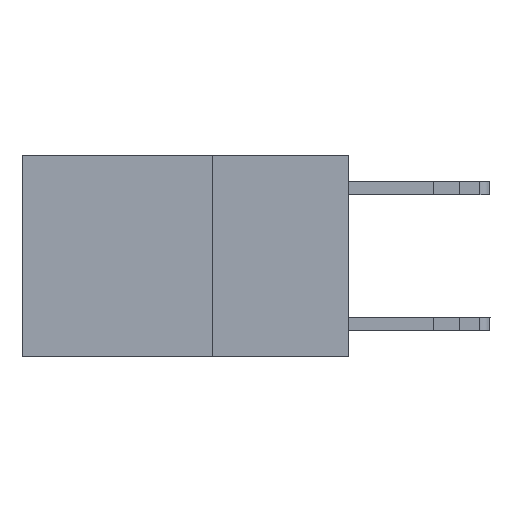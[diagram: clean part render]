
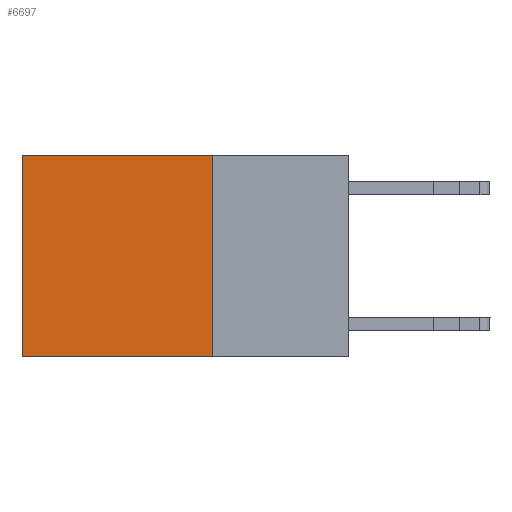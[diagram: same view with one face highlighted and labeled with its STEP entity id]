
A CAD part, left-side view. The second image highlights one B-rep face of the part: STEP entity #6697.
In plain terms, the highlighted planar face has unit normal (-1, 0, 0).
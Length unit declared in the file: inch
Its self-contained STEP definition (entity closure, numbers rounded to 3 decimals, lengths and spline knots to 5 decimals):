
#104 = DIRECTION ( 'NONE',  ( 0., 0., -1. ) ) ;
#108 = DIRECTION ( 'NONE',  ( 1., 0., 0. ) ) ;
#169 = CARTESIAN_POINT ( 'NONE',  ( 0.2625, 0.25, 0. ) ) ;
#196 = PLANE ( 'NONE',  #20548 ) ;
#1776 = CARTESIAN_POINT ( 'NONE',  ( 0.2625, 0.25, -0.37 ) ) ;
#4650 = LINE ( 'NONE', #10828, #4730 ) ;
#4730 = VECTOR ( 'NONE', #10849, 39.37008 ) ;
#6697 = ADVANCED_FACE ( 'NONE', ( #16287 ), #196, .F. ) ;
#6836 = VERTEX_POINT ( 'NONE', #17824 ) ;
#7561 = LINE ( 'NONE', #11658, #7807 ) ;
#7807 = VECTOR ( 'NONE', #11794, 39.37008 ) ;
#7953 = VECTOR ( 'NONE', #23485, 39.37008 ) ;
#8127 = LINE ( 'NONE', #12548, #7953 ) ;
#8470 = EDGE_CURVE ( 'NONE', #11302, #6836, #4650, .T. ) ;
#9024 = EDGE_LOOP ( 'NONE', ( #9986, #10343, #18414, #11595 ) ) ;
#9986 = ORIENTED_EDGE ( 'NONE', *, *, #10537, .T. ) ;
#10343 = ORIENTED_EDGE ( 'NONE', *, *, #12279, .F. ) ;
#10537 = EDGE_CURVE ( 'NONE', #6836, #23952, #18042, .T. ) ;
#10828 = CARTESIAN_POINT ( 'NONE',  ( 0.2625, 0.25, 0. ) ) ;
#10849 = DIRECTION ( 'NONE',  ( 0., 1., 0. ) ) ;
#11302 = VERTEX_POINT ( 'NONE', #22841 ) ;
#11595 = ORIENTED_EDGE ( 'NONE', *, *, #8470, .T. ) ;
#11658 = CARTESIAN_POINT ( 'NONE',  ( 0.2625, 0.25, -0.37 ) ) ;
#11794 = DIRECTION ( 'NONE',  ( 0., 1., 0. ) ) ;
#12279 = EDGE_CURVE ( 'NONE', #14532, #23952, #7561, .T. ) ;
#12548 = CARTESIAN_POINT ( 'NONE',  ( 0.2625, 0.25, 0. ) ) ;
#14532 = VERTEX_POINT ( 'NONE', #1776 ) ;
#16287 = FACE_OUTER_BOUND ( 'NONE', #9024, .T. ) ;
#17824 = CARTESIAN_POINT ( 'NONE',  ( 0.2625, 0.6, 0. ) ) ;
#17949 = VECTOR ( 'NONE', #19482, 39.37008 ) ;
#18042 = LINE ( 'NONE', #19456, #17949 ) ;
#18414 = ORIENTED_EDGE ( 'NONE', *, *, #21695, .F. ) ;
#19456 = CARTESIAN_POINT ( 'NONE',  ( 0.2625, 0.6, 0. ) ) ;
#19482 = DIRECTION ( 'NONE',  ( 0., 0., -1. ) ) ;
#20548 = AXIS2_PLACEMENT_3D ( 'NONE', #169, #108, #104 ) ;
#21695 = EDGE_CURVE ( 'NONE', #11302, #14532, #8127, .T. ) ;
#22297 = CARTESIAN_POINT ( 'NONE',  ( 0.2625, 0.6, -0.37 ) ) ;
#22841 = CARTESIAN_POINT ( 'NONE',  ( 0.2625, 0.25, 0. ) ) ;
#23485 = DIRECTION ( 'NONE',  ( 0., 0., -1. ) ) ;
#23952 = VERTEX_POINT ( 'NONE', #22297 ) ;
